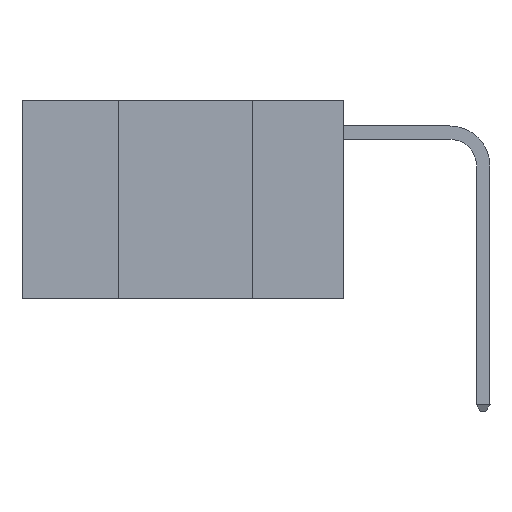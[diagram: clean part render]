
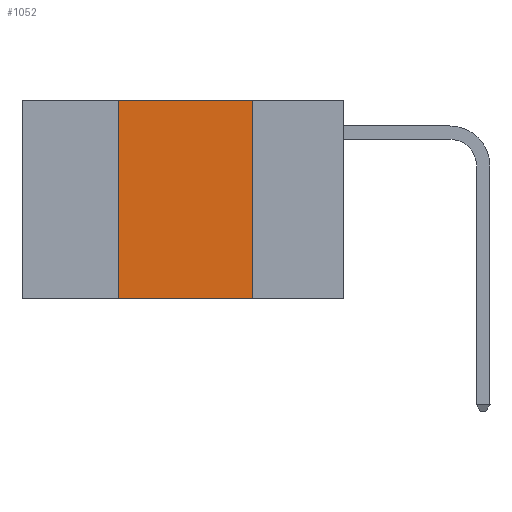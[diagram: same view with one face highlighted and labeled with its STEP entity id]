
A CAD part, left-side view. The second image highlights one B-rep face of the part: STEP entity #1052.
In plain terms, the highlighted planar face has unit normal (-1, 0, 0).
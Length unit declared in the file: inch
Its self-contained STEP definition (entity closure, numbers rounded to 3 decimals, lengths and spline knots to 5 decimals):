
#148 = VECTOR ( 'NONE', #8677, 39.37008 ) ;
#279 = ORIENTED_EDGE ( 'NONE', *, *, #3513, .T. ) ;
#791 = DIRECTION ( 'NONE',  ( 0., -1., 0. ) ) ;
#1052 = ADVANCED_FACE ( 'NONE', ( #1170 ), #4006, .F. ) ;
#1170 = FACE_OUTER_BOUND ( 'NONE', #6181, .T. ) ;
#1733 = DIRECTION ( 'NONE',  ( 0., -1., 0. ) ) ;
#2374 = LINE ( 'NONE', #8079, #7564 ) ;
#2732 = DIRECTION ( 'NONE',  ( 1., 0., 0. ) ) ;
#2930 = DIRECTION ( 'NONE',  ( 0., 0., -1. ) ) ;
#3146 = CARTESIAN_POINT ( 'NONE',  ( 0., 0.42, -0.37 ) ) ;
#3445 = LINE ( 'NONE', #8500, #7833 ) ;
#3501 = ORIENTED_EDGE ( 'NONE', *, *, #5174, .F. ) ;
#3513 = EDGE_CURVE ( 'NONE', #6002, #8760, #4766, .T. ) ;
#3891 = ORIENTED_EDGE ( 'NONE', *, *, #4542, .F. ) ;
#4006 = PLANE ( 'NONE',  #5374 ) ;
#4424 = LINE ( 'NONE', #6726, #148 ) ;
#4542 = EDGE_CURVE ( 'NONE', #6002, #6961, #3445, .T. ) ;
#4585 = CARTESIAN_POINT ( 'NONE',  ( 0., 0.6, -0.37 ) ) ;
#4766 = LINE ( 'NONE', #4585, #8570 ) ;
#4847 = DIRECTION ( 'NONE',  ( 0., 0., 1. ) ) ;
#5174 = EDGE_CURVE ( 'NONE', #6961, #5921, #2374, .T. ) ;
#5374 = AXIS2_PLACEMENT_3D ( 'NONE', #7004, #2732, #2930 ) ;
#5799 = CARTESIAN_POINT ( 'NONE',  ( 0., 0.17, 0. ) ) ;
#5921 = VERTEX_POINT ( 'NONE', #5799 ) ;
#6002 = VERTEX_POINT ( 'NONE', #3146 ) ;
#6181 = EDGE_LOOP ( 'NONE', ( #8863, #3501, #3891, #279 ) ) ;
#6592 = CARTESIAN_POINT ( 'NONE',  ( 0., 0.42, 0. ) ) ;
#6726 = CARTESIAN_POINT ( 'NONE',  ( 0., 0.17, 0. ) ) ;
#6961 = VERTEX_POINT ( 'NONE', #6592 ) ;
#7004 = CARTESIAN_POINT ( 'NONE',  ( 0., 0.6, 0. ) ) ;
#7564 = VECTOR ( 'NONE', #791, 39.37008 ) ;
#7833 = VECTOR ( 'NONE', #4847, 39.37008 ) ;
#8079 = CARTESIAN_POINT ( 'NONE',  ( 0., 0.6, 0. ) ) ;
#8391 = CARTESIAN_POINT ( 'NONE',  ( 0., 0.17, -0.37 ) ) ;
#8500 = CARTESIAN_POINT ( 'NONE',  ( 0., 0.42, 0. ) ) ;
#8570 = VECTOR ( 'NONE', #1733, 39.37008 ) ;
#8635 = EDGE_CURVE ( 'NONE', #5921, #8760, #4424, .T. ) ;
#8677 = DIRECTION ( 'NONE',  ( 0., 0., -1. ) ) ;
#8760 = VERTEX_POINT ( 'NONE', #8391 ) ;
#8863 = ORIENTED_EDGE ( 'NONE', *, *, #8635, .F. ) ;
